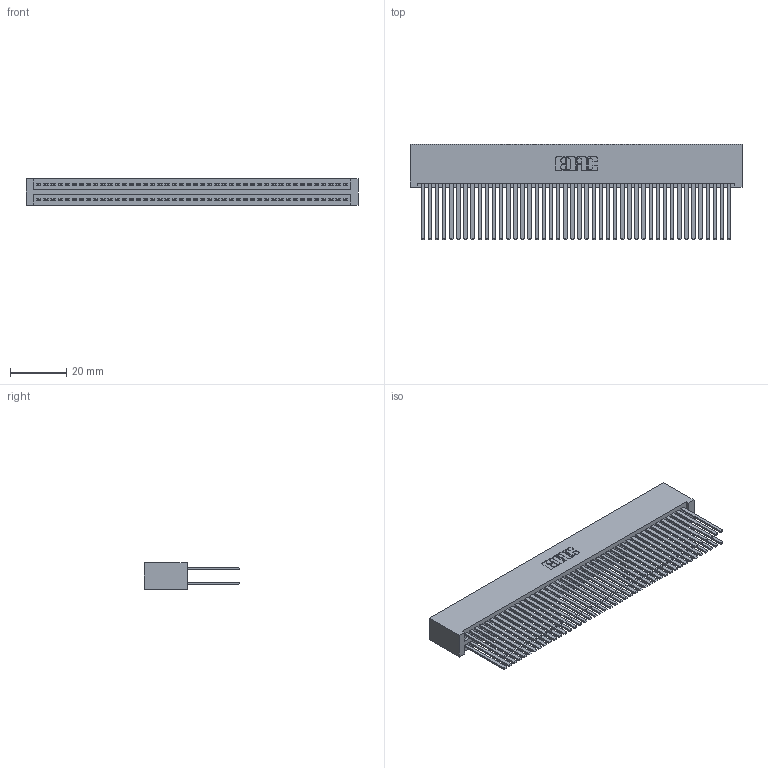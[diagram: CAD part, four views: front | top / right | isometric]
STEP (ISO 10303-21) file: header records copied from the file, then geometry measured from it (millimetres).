
FILE_DESCRIPTION (( 'STEP AP203' ), '1' );
FILE_NAME ('345-088-544-201.STEP', '2018-10-04T14:14:18', ( '' ), ( '' ), 'SwSTEP 2.0', 'SolidWorks 2016', '' );
FILE_SCHEMA (( 'CONFIG_CONTROL_DESIGN' ));
Length unit declared in the file: inch
Products named in the file (3): 345-088-544-201; 345-292-001_345-293-144; 345 Part_No Mounting Lugs
Assembly tree (89 placements, depth 2):
  345-088-544-201
    345 Part_No Mounting Lugs
    345-292-001_345-293-144  x88
Bounding box: 118.36 x 33.96 x 9.4 mm (x, y, z)
Volume: 13366.1 mm3; surface area: 23714.9 mm2
Topology: 89 solids, 89 shells, 3990 faces, 11845 edges, 7778 vertices
Faces by surface type: plane 2628, cylinder 1362
Entity records: 33793 total; most frequent: CARTESIAN_POINT 5660, ORIENTED_EDGE 5594, DIRECTION 4981, EDGE_CURVE 2797, VECTOR 2501, LINE 2501, VERTEX_POINT 1862, AXIS2_PLACEMENT_3D 1240
